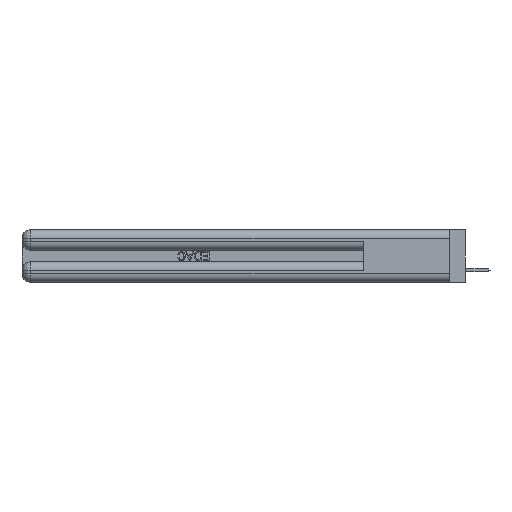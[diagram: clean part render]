
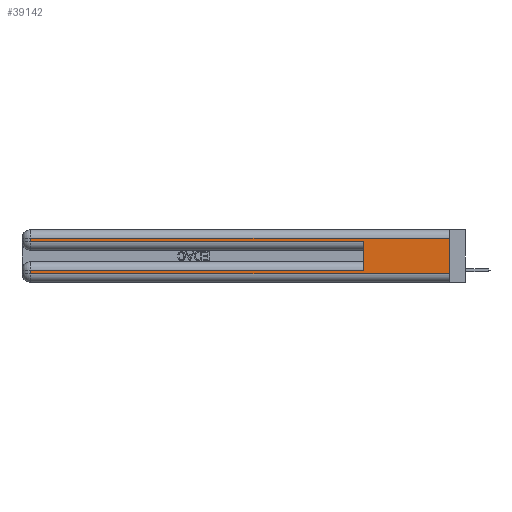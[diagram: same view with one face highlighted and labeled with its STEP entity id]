
A CAD part, left-side view. The second image highlights one B-rep face of the part: STEP entity #39142.
In plain terms, the highlighted planar face has unit normal (-1, 0, 0).
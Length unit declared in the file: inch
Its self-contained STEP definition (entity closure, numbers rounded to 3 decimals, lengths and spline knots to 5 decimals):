
#39 = VERTEX_POINT ( 'NONE', #6244 ) ;
#1088 = CARTESIAN_POINT ( 'NONE',  ( 0., 0., 0.06 ) ) ;
#1216 = EDGE_CURVE ( 'NONE', #14898, #32346, #26409, .T. ) ;
#4123 = EDGE_CURVE ( 'NONE', #14898, #39, #49563, .T. ) ;
#4417 = DIRECTION ( 'NONE',  ( 0., 0., -1. ) ) ;
#4640 = CARTESIAN_POINT ( 'NONE',  ( 0., 0., 0.285 ) ) ;
#5483 = DIRECTION ( 'NONE',  ( 0., 1., 0. ) ) ;
#5502 = ORIENTED_EDGE ( 'NONE', *, *, #32740, .T. ) ;
#6244 = CARTESIAN_POINT ( 'NONE',  ( 0., 2.94, 0.085 ) ) ;
#7176 = LINE ( 'NONE', #37561, #47991 ) ;
#7492 = VECTOR ( 'NONE', #5483, 39.37008 ) ;
#7516 = CARTESIAN_POINT ( 'NONE',  ( 0., 0.6, 0.285 ) ) ;
#8441 = EDGE_LOOP ( 'NONE', ( #29498, #5502, #16313, #47798, #18600, #44169, #14961, #29814 ) ) ;
#9627 = CARTESIAN_POINT ( 'NONE',  ( 0., 2.94, 0.31 ) ) ;
#10051 = DIRECTION ( 'NONE',  ( 0., 1., 0. ) ) ;
#11298 = EDGE_CURVE ( 'NONE', #39, #31111, #15663, .T. ) ;
#11330 = EDGE_CURVE ( 'NONE', #14566, #32346, #12537, .T. ) ;
#11935 = CARTESIAN_POINT ( 'NONE',  ( 0., 0., 0.06 ) ) ;
#12537 = LINE ( 'NONE', #4640, #31171 ) ;
#14566 = VERTEX_POINT ( 'NONE', #28857 ) ;
#14898 = VERTEX_POINT ( 'NONE', #19771 ) ;
#14961 = ORIENTED_EDGE ( 'NONE', *, *, #11298, .T. ) ;
#15493 = DIRECTION ( 'NONE',  ( 0., 0., -1. ) ) ;
#15539 = CARTESIAN_POINT ( 'NONE',  ( 0., 0., 0.37 ) ) ;
#15655 = VERTEX_POINT ( 'NONE', #17924 ) ;
#15663 = LINE ( 'NONE', #43681, #36149 ) ;
#16313 = ORIENTED_EDGE ( 'NONE', *, *, #38938, .T. ) ;
#17657 = FACE_OUTER_BOUND ( 'NONE', #8441, .T. ) ;
#17924 = CARTESIAN_POINT ( 'NONE',  ( 0., 0., 0.31 ) ) ;
#18600 = ORIENTED_EDGE ( 'NONE', *, *, #1216, .F. ) ;
#19492 = PLANE ( 'NONE',  #23173 ) ;
#19771 = CARTESIAN_POINT ( 'NONE',  ( 0., 0.6, 0.085 ) ) ;
#20514 = VERTEX_POINT ( 'NONE', #9627 ) ;
#21085 = DIRECTION ( 'NONE',  ( 0., 0., -1. ) ) ;
#21298 = VERTEX_POINT ( 'NONE', #11935 ) ;
#22857 = DIRECTION ( 'NONE',  ( 0., 0., -1. ) ) ;
#23173 = AXIS2_PLACEMENT_3D ( 'NONE', #15539, #34964, #22857 ) ;
#23619 = VECTOR ( 'NONE', #10051, 39.37008 ) ;
#24516 = VECTOR ( 'NONE', #41382, 39.37008 ) ;
#24610 = DIRECTION ( 'NONE',  ( 0., -1., 0. ) ) ;
#25663 = EDGE_CURVE ( 'NONE', #31111, #21298, #27582, .T. ) ;
#26409 = LINE ( 'NONE', #46674, #24516 ) ;
#27582 = LINE ( 'NONE', #1088, #30642 ) ;
#27882 = CARTESIAN_POINT ( 'NONE',  ( 0., 2.94, 0.06 ) ) ;
#28857 = CARTESIAN_POINT ( 'NONE',  ( 0., 2.94, 0.285 ) ) ;
#29498 = ORIENTED_EDGE ( 'NONE', *, *, #50274, .F. ) ;
#29666 = CARTESIAN_POINT ( 'NONE',  ( 0., 0., 0.31 ) ) ;
#29814 = ORIENTED_EDGE ( 'NONE', *, *, #25663, .T. ) ;
#30642 = VECTOR ( 'NONE', #36832, 39.37008 ) ;
#31111 = VERTEX_POINT ( 'NONE', #27882 ) ;
#31171 = VECTOR ( 'NONE', #24610, 39.37008 ) ;
#32294 = LINE ( 'NONE', #29666, #23619 ) ;
#32346 = VERTEX_POINT ( 'NONE', #7516 ) ;
#32740 = EDGE_CURVE ( 'NONE', #15655, #20514, #32294, .T. ) ;
#34964 = DIRECTION ( 'NONE',  ( 1., 0., 0. ) ) ;
#36149 = VECTOR ( 'NONE', #4417, 39.37008 ) ;
#36832 = DIRECTION ( 'NONE',  ( 0., -1., 0. ) ) ;
#37561 = CARTESIAN_POINT ( 'NONE',  ( 0., 2.94, 0.37 ) ) ;
#38938 = EDGE_CURVE ( 'NONE', #20514, #14566, #7176, .T. ) ;
#39142 = ADVANCED_FACE ( 'NONE', ( #17657 ), #19492, .F. ) ;
#41382 = DIRECTION ( 'NONE',  ( 0., 0., 1. ) ) ;
#41609 = LINE ( 'NONE', #51255, #50797 ) ;
#43681 = CARTESIAN_POINT ( 'NONE',  ( 0., 2.94, 0.37 ) ) ;
#44169 = ORIENTED_EDGE ( 'NONE', *, *, #4123, .T. ) ;
#46674 = CARTESIAN_POINT ( 'NONE',  ( 0., 0.6, 0.145 ) ) ;
#47798 = ORIENTED_EDGE ( 'NONE', *, *, #11330, .T. ) ;
#47991 = VECTOR ( 'NONE', #21085, 39.37008 ) ;
#48537 = CARTESIAN_POINT ( 'NONE',  ( 0., 0., 0.085 ) ) ;
#49563 = LINE ( 'NONE', #48537, #7492 ) ;
#50274 = EDGE_CURVE ( 'NONE', #15655, #21298, #41609, .T. ) ;
#50797 = VECTOR ( 'NONE', #15493, 39.37008 ) ;
#51255 = CARTESIAN_POINT ( 'NONE',  ( 0., 0., 0.37 ) ) ;
